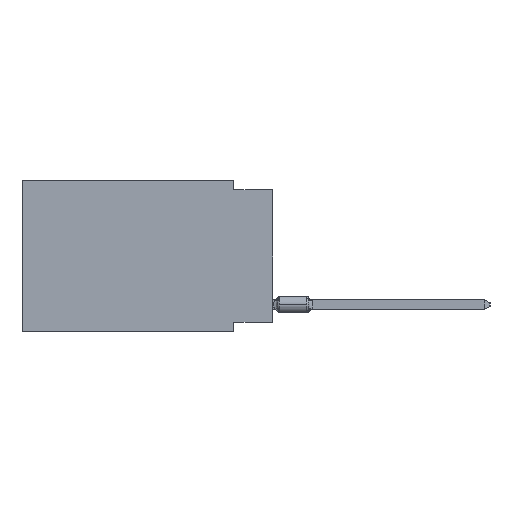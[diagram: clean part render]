
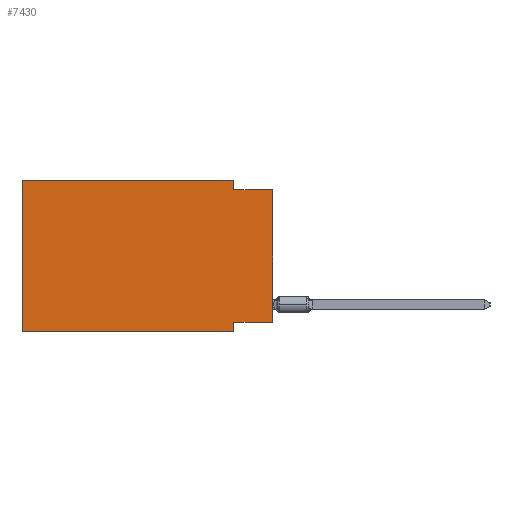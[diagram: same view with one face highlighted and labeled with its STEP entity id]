
A CAD part, left-side view. The second image highlights one B-rep face of the part: STEP entity #7430.
In plain terms, the highlighted planar face has unit normal (-1, 0, 0).
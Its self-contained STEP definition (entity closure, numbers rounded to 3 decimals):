
#413 = LINE ( 'NONE', #24279, #5120 ) ;
#499 = DIRECTION ( 'NONE',  ( 0., 0., -1. ) ) ;
#589 = EDGE_CURVE ( 'NONE', #19620, #27727, #42715, .T. ) ;
#704 = CARTESIAN_POINT ( 'NONE',  ( 0., 16.383, 0. ) ) ;
#2722 = LINE ( 'NONE', #63339, #58998 ) ;
#5120 = VECTOR ( 'NONE', #19037, 1000. ) ;
#6570 = DIRECTION ( 'NONE',  ( 1., 0., 0. ) ) ;
#7430 = ADVANCED_FACE ( 'NONE', ( #12655 ), #50605, .F. ) ;
#12655 = FACE_OUTER_BOUND ( 'NONE', #66612, .T. ) ;
#15611 = CARTESIAN_POINT ( 'NONE',  ( 0., 0., -9.271 ) ) ;
#17695 = LINE ( 'NONE', #24930, #60793 ) ;
#18082 = DIRECTION ( 'NONE',  ( 0., -1., 0. ) ) ;
#18197 = ORIENTED_EDGE ( 'NONE', *, *, #23282, .F. ) ;
#19037 = DIRECTION ( 'NONE',  ( 0., 0., 1. ) ) ;
#19045 = CARTESIAN_POINT ( 'NONE',  ( 0., 0., -9.271 ) ) ;
#19620 = VERTEX_POINT ( 'NONE', #62480 ) ;
#20114 = ORIENTED_EDGE ( 'NONE', *, *, #31947, .T. ) ;
#20422 = DIRECTION ( 'NONE',  ( 0., -1., 0. ) ) ;
#20540 = VECTOR ( 'NONE', #20422, 1000. ) ;
#20766 = CARTESIAN_POINT ( 'NONE',  ( 0., 2.54, 0. ) ) ;
#22368 = CARTESIAN_POINT ( 'NONE',  ( 0., 2.54, -9.271 ) ) ;
#23282 = EDGE_CURVE ( 'NONE', #68599, #33483, #38128, .T. ) ;
#24279 = CARTESIAN_POINT ( 'NONE',  ( 0., 16.383, 0. ) ) ;
#24930 = CARTESIAN_POINT ( 'NONE',  ( 0., 2.54, -9.906 ) ) ;
#26041 = ORIENTED_EDGE ( 'NONE', *, *, #32812, .F. ) ;
#26045 = ORIENTED_EDGE ( 'NONE', *, *, #77648, .F. ) ;
#26742 = CARTESIAN_POINT ( 'NONE',  ( 0., 2.54, -0.635 ) ) ;
#26875 = LINE ( 'NONE', #704, #20540 ) ;
#27727 = VERTEX_POINT ( 'NONE', #31813 ) ;
#30872 = VECTOR ( 'NONE', #53783, 1000. ) ;
#31813 = CARTESIAN_POINT ( 'NONE',  ( 0., 2.54, -9.906 ) ) ;
#31947 = EDGE_CURVE ( 'NONE', #39280, #41853, #2722, .T. ) ;
#32070 = DIRECTION ( 'NONE',  ( 0., 0., -1. ) ) ;
#32812 = EDGE_CURVE ( 'NONE', #39280, #51992, #53541, .T. ) ;
#32895 = ORIENTED_EDGE ( 'NONE', *, *, #589, .T. ) ;
#33483 = VERTEX_POINT ( 'NONE', #26742 ) ;
#34479 = ORIENTED_EDGE ( 'NONE', *, *, #38039, .F. ) ;
#35440 = EDGE_CURVE ( 'NONE', #36470, #68599, #26875, .T. ) ;
#36395 = LINE ( 'NONE', #78816, #30872 ) ;
#36470 = VERTEX_POINT ( 'NONE', #63116 ) ;
#38039 = EDGE_CURVE ( 'NONE', #19620, #36470, #413, .T. ) ;
#38128 = LINE ( 'NONE', #20766, #45148 ) ;
#38476 = CARTESIAN_POINT ( 'NONE',  ( 0., 16.383, 0. ) ) ;
#39280 = VERTEX_POINT ( 'NONE', #19045 ) ;
#40072 = CARTESIAN_POINT ( 'NONE',  ( 0., 2.54, 0. ) ) ;
#41853 = VERTEX_POINT ( 'NONE', #53404 ) ;
#42715 = LINE ( 'NONE', #67361, #44976 ) ;
#43113 = DIRECTION ( 'NONE',  ( 0., 0., -1. ) ) ;
#44976 = VECTOR ( 'NONE', #18082, 1000. ) ;
#45148 = VECTOR ( 'NONE', #32070, 1000. ) ;
#50605 = PLANE ( 'NONE',  #69043 ) ;
#51319 = VECTOR ( 'NONE', #77785, 1000. ) ;
#51666 = ORIENTED_EDGE ( 'NONE', *, *, #66565, .F. ) ;
#51992 = VERTEX_POINT ( 'NONE', #22368 ) ;
#53404 = CARTESIAN_POINT ( 'NONE',  ( 0., 0., -0.635 ) ) ;
#53541 = LINE ( 'NONE', #15611, #51319 ) ;
#53783 = DIRECTION ( 'NONE',  ( 0., -1., 0. ) ) ;
#58085 = DIRECTION ( 'NONE',  ( 0., 0., 1. ) ) ;
#58998 = VECTOR ( 'NONE', #58085, 1000. ) ;
#60793 = VECTOR ( 'NONE', #43113, 1000. ) ;
#62480 = CARTESIAN_POINT ( 'NONE',  ( 0., 16.383, -9.906 ) ) ;
#63116 = CARTESIAN_POINT ( 'NONE',  ( 0., 16.383, 0. ) ) ;
#63339 = CARTESIAN_POINT ( 'NONE',  ( 0., 0., 0. ) ) ;
#66565 = EDGE_CURVE ( 'NONE', #33483, #41853, #36395, .T. ) ;
#66612 = EDGE_LOOP ( 'NONE', ( #20114, #51666, #18197, #74713, #34479, #32895, #26045, #26041 ) ) ;
#67361 = CARTESIAN_POINT ( 'NONE',  ( 0., 16.383, -9.906 ) ) ;
#68599 = VERTEX_POINT ( 'NONE', #40072 ) ;
#69043 = AXIS2_PLACEMENT_3D ( 'NONE', #38476, #6570, #499 ) ;
#74713 = ORIENTED_EDGE ( 'NONE', *, *, #35440, .F. ) ;
#77648 = EDGE_CURVE ( 'NONE', #51992, #27727, #17695, .T. ) ;
#77785 = DIRECTION ( 'NONE',  ( 0., 1., 0. ) ) ;
#78816 = CARTESIAN_POINT ( 'NONE',  ( 0., 0., -0.635 ) ) ;
